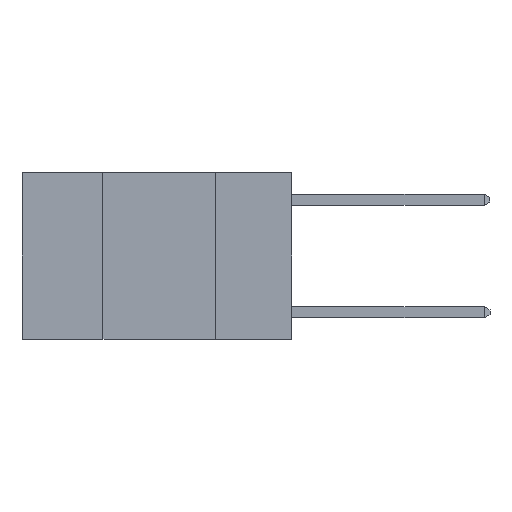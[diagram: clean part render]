
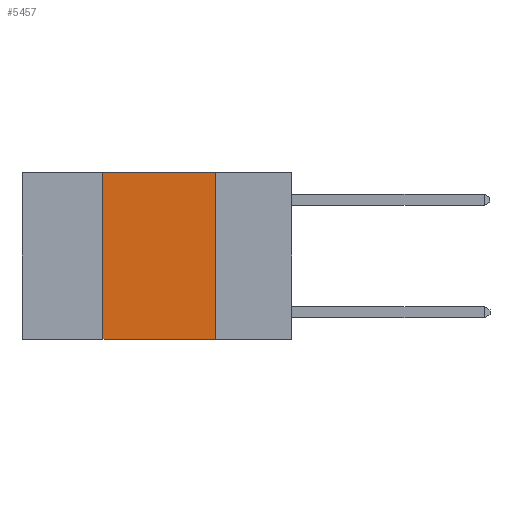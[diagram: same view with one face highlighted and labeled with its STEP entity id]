
A CAD part, left-side view. The second image highlights one B-rep face of the part: STEP entity #5457.
In plain terms, the highlighted planar face has unit normal (-1, 0, 0).
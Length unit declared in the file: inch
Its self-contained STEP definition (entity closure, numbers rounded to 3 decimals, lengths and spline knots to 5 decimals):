
#408 = FACE_OUTER_BOUND ( 'NONE', #8717, .T. ) ;
#684 = LINE ( 'NONE', #10096, #6204 ) ;
#1173 = CARTESIAN_POINT ( 'NONE',  ( 0., 0.17, 0. ) ) ;
#1353 = DIRECTION ( 'NONE',  ( 0., 0., -1. ) ) ;
#1450 = VECTOR ( 'NONE', #1353, 39.37008 ) ;
#1908 = VERTEX_POINT ( 'NONE', #6984 ) ;
#2073 = LINE ( 'NONE', #7751, #6209 ) ;
#2467 = EDGE_CURVE ( 'NONE', #10109, #1908, #684, .T. ) ;
#2666 = VERTEX_POINT ( 'NONE', #5345 ) ;
#2789 = DIRECTION ( 'NONE',  ( 0., 0., 1. ) ) ;
#3004 = VECTOR ( 'NONE', #4300, 39.37008 ) ;
#3178 = CARTESIAN_POINT ( 'NONE',  ( 0., 0.17, -0.37 ) ) ;
#3272 = DIRECTION ( 'NONE',  ( 1., 0., 0. ) ) ;
#3499 = CARTESIAN_POINT ( 'NONE',  ( 0., 0.42, 0. ) ) ;
#3697 = EDGE_CURVE ( 'NONE', #1908, #8198, #8046, .T. ) ;
#4068 = CARTESIAN_POINT ( 'NONE',  ( 0., 0.6, 0. ) ) ;
#4300 = DIRECTION ( 'NONE',  ( 0., -1., 0. ) ) ;
#5024 = EDGE_CURVE ( 'NONE', #2666, #10109, #2073, .T. ) ;
#5205 = LINE ( 'NONE', #9243, #3004 ) ;
#5345 = CARTESIAN_POINT ( 'NONE',  ( 0., 0.42, -0.37 ) ) ;
#5457 = ADVANCED_FACE ( 'NONE', ( #408 ), #6584, .F. ) ;
#5555 = ORIENTED_EDGE ( 'NONE', *, *, #3697, .F. ) ;
#6204 = VECTOR ( 'NONE', #6560, 39.37008 ) ;
#6209 = VECTOR ( 'NONE', #2789, 39.37008 ) ;
#6560 = DIRECTION ( 'NONE',  ( 0., -1., 0. ) ) ;
#6584 = PLANE ( 'NONE',  #7638 ) ;
#6984 = CARTESIAN_POINT ( 'NONE',  ( 0., 0.17, 0. ) ) ;
#7128 = ORIENTED_EDGE ( 'NONE', *, *, #5024, .F. ) ;
#7638 = AXIS2_PLACEMENT_3D ( 'NONE', #4068, #3272, #9058 ) ;
#7751 = CARTESIAN_POINT ( 'NONE',  ( 0., 0.42, 0. ) ) ;
#8046 = LINE ( 'NONE', #1173, #1450 ) ;
#8198 = VERTEX_POINT ( 'NONE', #3178 ) ;
#8717 = EDGE_LOOP ( 'NONE', ( #5555, #9047, #7128, #9194 ) ) ;
#8892 = EDGE_CURVE ( 'NONE', #2666, #8198, #5205, .T. ) ;
#9047 = ORIENTED_EDGE ( 'NONE', *, *, #2467, .F. ) ;
#9058 = DIRECTION ( 'NONE',  ( 0., 0., -1. ) ) ;
#9194 = ORIENTED_EDGE ( 'NONE', *, *, #8892, .T. ) ;
#9243 = CARTESIAN_POINT ( 'NONE',  ( 0., 0.6, -0.37 ) ) ;
#10096 = CARTESIAN_POINT ( 'NONE',  ( 0., 0.6, 0. ) ) ;
#10109 = VERTEX_POINT ( 'NONE', #3499 ) ;
